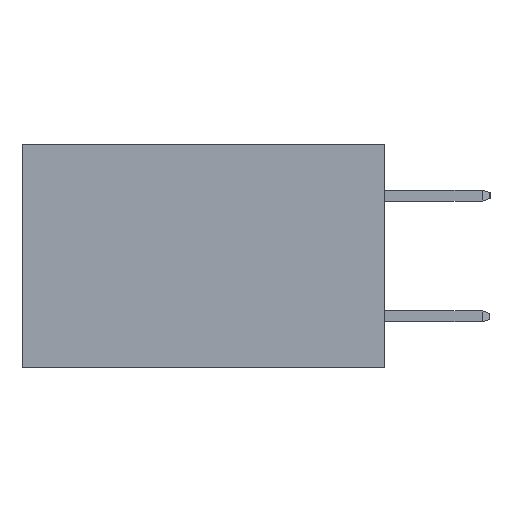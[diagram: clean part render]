
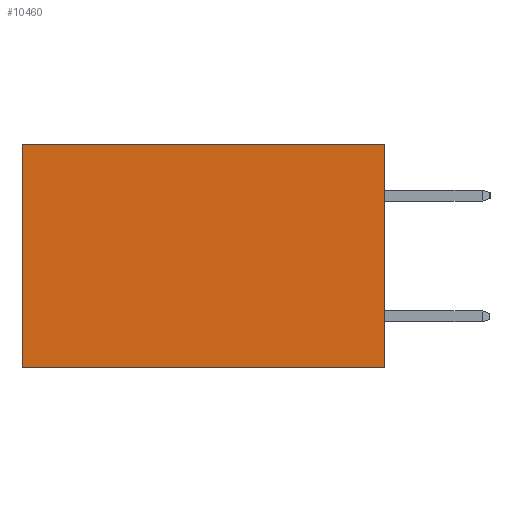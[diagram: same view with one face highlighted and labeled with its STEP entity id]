
A CAD part, left-side view. The second image highlights one B-rep face of the part: STEP entity #10460.
In plain terms, the highlighted planar face has unit normal (-1, 0, 0).
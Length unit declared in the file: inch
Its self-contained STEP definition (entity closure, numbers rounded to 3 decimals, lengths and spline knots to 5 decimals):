
#128 = DIRECTION ( 'NONE',  ( 0., 0., -1. ) ) ;
#147 = DIRECTION ( 'NONE',  ( 1., 0., 0. ) ) ;
#184 = CARTESIAN_POINT ( 'NONE',  ( 0.298, 0., 0. ) ) ;
#197 = PLANE ( 'NONE',  #9045 ) ;
#1012 = DIRECTION ( 'NONE',  ( 0., 1., 0. ) ) ;
#1114 = EDGE_CURVE ( 'NONE', #7574, #8948, #12542, .T. ) ;
#1307 = VECTOR ( 'NONE', #6842, 39.37008 ) ;
#1475 = CARTESIAN_POINT ( 'NONE',  ( 0.298, 0.6, 0. ) ) ;
#1912 = ORIENTED_EDGE ( 'NONE', *, *, #1114, .F. ) ;
#2403 = VECTOR ( 'NONE', #8652, 39.37008 ) ;
#2410 = EDGE_CURVE ( 'NONE', #8948, #11479, #8255, .T. ) ;
#2654 = VECTOR ( 'NONE', #1012, 39.37008 ) ;
#3322 = FACE_OUTER_BOUND ( 'NONE', #12253, .T. ) ;
#4246 = CARTESIAN_POINT ( 'NONE',  ( 0.298, 0., 0. ) ) ;
#5284 = EDGE_CURVE ( 'NONE', #7987, #11479, #15377, .T. ) ;
#5314 = ORIENTED_EDGE ( 'NONE', *, *, #5284, .T. ) ;
#5892 = VECTOR ( 'NONE', #7334, 39.37008 ) ;
#6145 = LINE ( 'NONE', #16057, #2654 ) ;
#6842 = DIRECTION ( 'NONE',  ( 0., 1., 0. ) ) ;
#7334 = DIRECTION ( 'NONE',  ( 0., 0., -1. ) ) ;
#7574 = VERTEX_POINT ( 'NONE', #4246 ) ;
#7987 = VERTEX_POINT ( 'NONE', #1475 ) ;
#8255 = LINE ( 'NONE', #12694, #1307 ) ;
#8501 = CARTESIAN_POINT ( 'NONE',  ( 0.298, 0.6, 0. ) ) ;
#8652 = DIRECTION ( 'NONE',  ( 0., 0., -1. ) ) ;
#8948 = VERTEX_POINT ( 'NONE', #14339 ) ;
#9045 = AXIS2_PLACEMENT_3D ( 'NONE', #184, #147, #128 ) ;
#9786 = ORIENTED_EDGE ( 'NONE', *, *, #15188, .T. ) ;
#10457 = CARTESIAN_POINT ( 'NONE',  ( 0.298, 0., 0. ) ) ;
#10460 = ADVANCED_FACE ( 'NONE', ( #3322 ), #197, .F. ) ;
#11479 = VERTEX_POINT ( 'NONE', #13885 ) ;
#12253 = EDGE_LOOP ( 'NONE', ( #5314, #12679, #1912, #9786 ) ) ;
#12542 = LINE ( 'NONE', #10457, #2403 ) ;
#12679 = ORIENTED_EDGE ( 'NONE', *, *, #2410, .F. ) ;
#12694 = CARTESIAN_POINT ( 'NONE',  ( 0.298, 0., -0.37 ) ) ;
#13885 = CARTESIAN_POINT ( 'NONE',  ( 0.298, 0.6, -0.37 ) ) ;
#14339 = CARTESIAN_POINT ( 'NONE',  ( 0.298, 0., -0.37 ) ) ;
#15188 = EDGE_CURVE ( 'NONE', #7574, #7987, #6145, .T. ) ;
#15377 = LINE ( 'NONE', #8501, #5892 ) ;
#16057 = CARTESIAN_POINT ( 'NONE',  ( 0.298, 0., 0. ) ) ;
